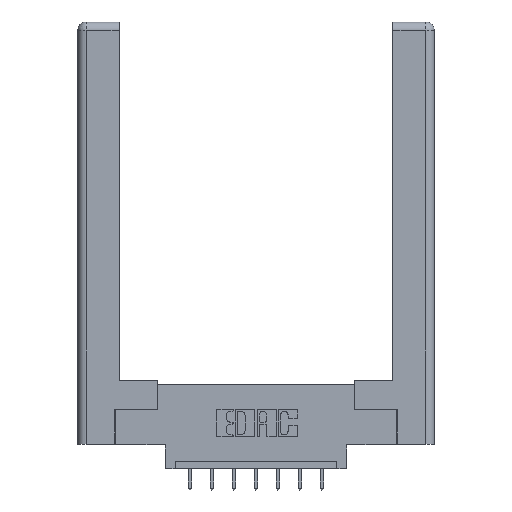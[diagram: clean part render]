
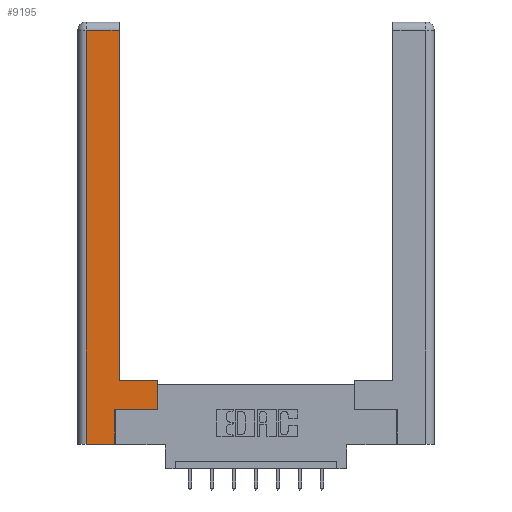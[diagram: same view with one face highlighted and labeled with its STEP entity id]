
A CAD part, top view. The second image highlights one B-rep face of the part: STEP entity #9195.
In plain terms, the highlighted planar face has unit normal (0, 0, 1).
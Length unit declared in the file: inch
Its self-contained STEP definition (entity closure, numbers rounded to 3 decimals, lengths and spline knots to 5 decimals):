
#90 = VECTOR ( 'NONE', #2884, 39.37008 ) ;
#393 = CARTESIAN_POINT ( 'NONE',  ( 0.0615, 0., 0. ) ) ;
#436 = DIRECTION ( 'NONE',  ( 1., 0., 0. ) ) ;
#483 = CARTESIAN_POINT ( 'NONE',  ( 0., 0., 0. ) ) ;
#672 = CARTESIAN_POINT ( 'NONE',  ( 0.565, 0.45, 0. ) ) ;
#1103 = ORIENTED_EDGE ( 'NONE', *, *, #6266, .T. ) ;
#1182 = CARTESIAN_POINT ( 'NONE',  ( 0.265, 0., 0. ) ) ;
#1592 = CARTESIAN_POINT ( 'NONE',  ( 0.295, 3., 0. ) ) ;
#1664 = VECTOR ( 'NONE', #7189, 39.37008 ) ;
#1691 = EDGE_CURVE ( 'NONE', #2194, #2169, #4817, .T. ) ;
#1846 = VECTOR ( 'NONE', #436, 39.37008 ) ;
#2169 = VERTEX_POINT ( 'NONE', #3545 ) ;
#2194 = VERTEX_POINT ( 'NONE', #9683 ) ;
#2351 = VECTOR ( 'NONE', #7197, 39.37008 ) ;
#2418 = VECTOR ( 'NONE', #9328, 39.37008 ) ;
#2806 = LINE ( 'NONE', #11585, #90 ) ;
#2884 = DIRECTION ( 'NONE',  ( 0., 1., 0. ) ) ;
#3179 = CARTESIAN_POINT ( 'NONE',  ( 0.295, 2.94, 0. ) ) ;
#3417 = CARTESIAN_POINT ( 'NONE',  ( 0.265, 0.245, 0. ) ) ;
#3452 = EDGE_CURVE ( 'NONE', #2169, #5543, #2806, .T. ) ;
#3481 = VECTOR ( 'NONE', #11450, 39.37008 ) ;
#3539 = EDGE_CURVE ( 'NONE', #10551, #2194, #7082, .T. ) ;
#3545 = CARTESIAN_POINT ( 'NONE',  ( 0.265, 0., 0. ) ) ;
#3583 = ORIENTED_EDGE ( 'NONE', *, *, #7230, .T. ) ;
#3649 = VERTEX_POINT ( 'NONE', #4530 ) ;
#4085 = LINE ( 'NONE', #1592, #1664 ) ;
#4392 = DIRECTION ( 'NONE',  ( 0., 0., -1. ) ) ;
#4426 = ORIENTED_EDGE ( 'NONE', *, *, #3452, .T. ) ;
#4530 = CARTESIAN_POINT ( 'NONE',  ( 0.295, 0.45, 0. ) ) ;
#4590 = CARTESIAN_POINT ( 'NONE',  ( 0.295, 0.45, 0. ) ) ;
#4776 = ORIENTED_EDGE ( 'NONE', *, *, #3539, .T. ) ;
#4817 = LINE ( 'NONE', #1182, #12411 ) ;
#4903 = EDGE_CURVE ( 'NONE', #5543, #11928, #9924, .T. ) ;
#5006 = CARTESIAN_POINT ( 'NONE',  ( 0.565, 0.245, 0. ) ) ;
#5310 = DIRECTION ( 'NONE',  ( -1., 0., 0. ) ) ;
#5375 = ORIENTED_EDGE ( 'NONE', *, *, #1691, .T. ) ;
#5428 = PLANE ( 'NONE',  #12051 ) ;
#5483 = CARTESIAN_POINT ( 'NONE',  ( 0.565, 0.45, 0. ) ) ;
#5543 = VERTEX_POINT ( 'NONE', #3417 ) ;
#5590 = LINE ( 'NONE', #672, #2418 ) ;
#6266 = EDGE_CURVE ( 'NONE', #9144, #10551, #6848, .T. ) ;
#6580 = VERTEX_POINT ( 'NONE', #5483 ) ;
#6847 = FACE_OUTER_BOUND ( 'NONE', #8875, .T. ) ;
#6848 = LINE ( 'NONE', #7481, #3481 ) ;
#6870 = EDGE_CURVE ( 'NONE', #3649, #9144, #4085, .T. ) ;
#7082 = LINE ( 'NONE', #393, #2351 ) ;
#7162 = EDGE_CURVE ( 'NONE', #11928, #6580, #5590, .T. ) ;
#7189 = DIRECTION ( 'NONE',  ( 0., 1., 0. ) ) ;
#7197 = DIRECTION ( 'NONE',  ( 0., -1., 0. ) ) ;
#7230 = EDGE_CURVE ( 'NONE', #6580, #3649, #9878, .T. ) ;
#7481 = CARTESIAN_POINT ( 'NONE',  ( 0.0615, 2.94, 0. ) ) ;
#8143 = DIRECTION ( 'NONE',  ( 1., 0., 0. ) ) ;
#8169 = ORIENTED_EDGE ( 'NONE', *, *, #4903, .T. ) ;
#8227 = CARTESIAN_POINT ( 'NONE',  ( 0.0615, 2.94, 0. ) ) ;
#8832 = VECTOR ( 'NONE', #10505, 39.37008 ) ;
#8875 = EDGE_LOOP ( 'NONE', ( #10574, #1103, #4776, #5375, #4426, #8169, #12406, #3583 ) ) ;
#9144 = VERTEX_POINT ( 'NONE', #3179 ) ;
#9195 = ADVANCED_FACE ( 'NONE', ( #6847 ), #5428, .F. ) ;
#9328 = DIRECTION ( 'NONE',  ( 0., 1., 0. ) ) ;
#9683 = CARTESIAN_POINT ( 'NONE',  ( 0.0615, 0., 0. ) ) ;
#9878 = LINE ( 'NONE', #4590, #8832 ) ;
#9924 = LINE ( 'NONE', #10279, #1846 ) ;
#10279 = CARTESIAN_POINT ( 'NONE',  ( 0.565, 0.245, 0. ) ) ;
#10505 = DIRECTION ( 'NONE',  ( -1., 0., 0. ) ) ;
#10551 = VERTEX_POINT ( 'NONE', #8227 ) ;
#10574 = ORIENTED_EDGE ( 'NONE', *, *, #6870, .T. ) ;
#11450 = DIRECTION ( 'NONE',  ( -1., 0., 0. ) ) ;
#11585 = CARTESIAN_POINT ( 'NONE',  ( 0.265, 0.245, 0. ) ) ;
#11928 = VERTEX_POINT ( 'NONE', #5006 ) ;
#12051 = AXIS2_PLACEMENT_3D ( 'NONE', #483, #4392, #5310 ) ;
#12406 = ORIENTED_EDGE ( 'NONE', *, *, #7162, .T. ) ;
#12411 = VECTOR ( 'NONE', #8143, 39.37008 ) ;
